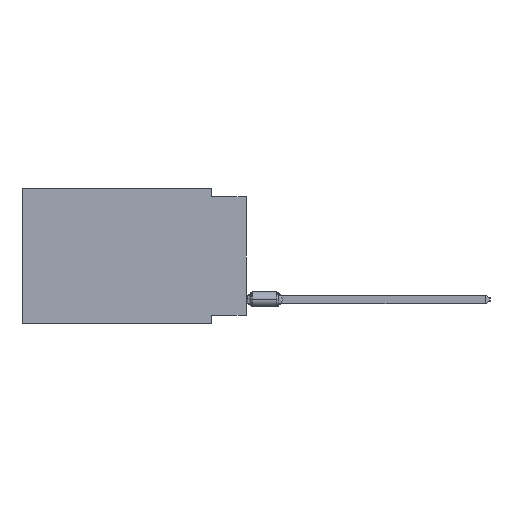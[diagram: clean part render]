
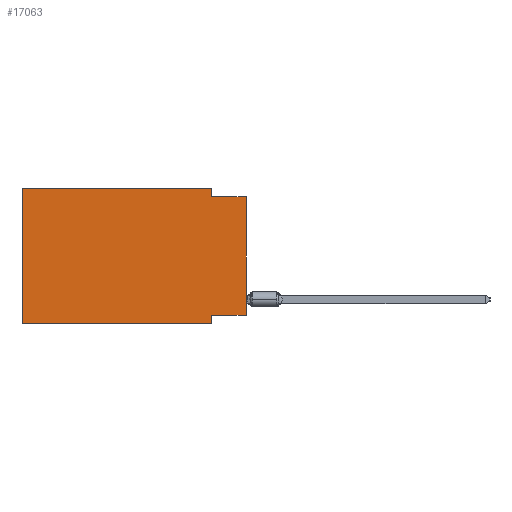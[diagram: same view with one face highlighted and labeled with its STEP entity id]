
A CAD part, left-side view. The second image highlights one B-rep face of the part: STEP entity #17063.
In plain terms, the highlighted planar face has unit normal (-1, 0, 0).
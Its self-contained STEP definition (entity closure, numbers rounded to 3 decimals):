
#175 = ORIENTED_EDGE ( 'NONE', *, *, #20337, .T. ) ;
#227 = CARTESIAN_POINT ( 'NONE',  ( 0., 2.54, 0. ) ) ;
#820 = LINE ( 'NONE', #16271, #21620 ) ;
#1589 = CARTESIAN_POINT ( 'NONE',  ( 0., 0., 0. ) ) ;
#2662 = CARTESIAN_POINT ( 'NONE',  ( 0., 16.383, 0. ) ) ;
#2813 = DIRECTION ( 'NONE',  ( 0., -1., 0. ) ) ;
#3084 = LINE ( 'NONE', #227, #20150 ) ;
#3428 = EDGE_LOOP ( 'NONE', ( #11187, #7930, #12192, #9831, #29777, #175, #21519, #31824 ) ) ;
#4492 = CARTESIAN_POINT ( 'NONE',  ( 0., 2.54, -0.635 ) ) ;
#5919 = DIRECTION ( 'NONE',  ( 0., 0., 1. ) ) ;
#6068 = LINE ( 'NONE', #15609, #21436 ) ;
#6574 = DIRECTION ( 'NONE',  ( 0., -1., 0. ) ) ;
#7838 = CARTESIAN_POINT ( 'NONE',  ( 0., 16.383, 0. ) ) ;
#7930 = ORIENTED_EDGE ( 'NONE', *, *, #35689, .F. ) ;
#8203 = VECTOR ( 'NONE', #6574, 1000. ) ;
#8391 = EDGE_CURVE ( 'NONE', #27628, #26745, #33743, .T. ) ;
#9180 = CARTESIAN_POINT ( 'NONE',  ( 0., 0., -9.271 ) ) ;
#9636 = LINE ( 'NONE', #22015, #8203 ) ;
#9831 = ORIENTED_EDGE ( 'NONE', *, *, #19126, .F. ) ;
#10632 = CARTESIAN_POINT ( 'NONE',  ( 0., 2.54, -9.906 ) ) ;
#11187 = ORIENTED_EDGE ( 'NONE', *, *, #39941, .T. ) ;
#11310 = PLANE ( 'NONE',  #29181 ) ;
#11545 = DIRECTION ( 'NONE',  ( 0., 0., -1. ) ) ;
#12192 = ORIENTED_EDGE ( 'NONE', *, *, #30972, .F. ) ;
#13540 = FACE_OUTER_BOUND ( 'NONE', #3428, .T. ) ;
#15276 = DIRECTION ( 'NONE',  ( 0., 0., -1. ) ) ;
#15609 = CARTESIAN_POINT ( 'NONE',  ( 0., 16.383, 0. ) ) ;
#15982 = EDGE_CURVE ( 'NONE', #39710, #19203, #22018, .T. ) ;
#16074 = VERTEX_POINT ( 'NONE', #36632 ) ;
#16271 = CARTESIAN_POINT ( 'NONE',  ( 0., 0., -0.635 ) ) ;
#16374 = VECTOR ( 'NONE', #5919, 1000. ) ;
#17063 = ADVANCED_FACE ( 'NONE', ( #13540 ), #11310, .F. ) ;
#17329 = VERTEX_POINT ( 'NONE', #4492 ) ;
#18979 = VERTEX_POINT ( 'NONE', #10632 ) ;
#19126 = EDGE_CURVE ( 'NONE', #26745, #16074, #6068, .T. ) ;
#19203 = VERTEX_POINT ( 'NONE', #38316 ) ;
#20150 = VECTOR ( 'NONE', #15276, 1000. ) ;
#20281 = DIRECTION ( 'NONE',  ( 0., 0., 1. ) ) ;
#20337 = EDGE_CURVE ( 'NONE', #27628, #18979, #9636, .T. ) ;
#20988 = CARTESIAN_POINT ( 'NONE',  ( 0., 16.383, -9.906 ) ) ;
#21436 = VECTOR ( 'NONE', #2813, 1000. ) ;
#21519 = ORIENTED_EDGE ( 'NONE', *, *, #37489, .F. ) ;
#21620 = VECTOR ( 'NONE', #22365, 1000. ) ;
#22015 = CARTESIAN_POINT ( 'NONE',  ( 0., 16.383, -9.906 ) ) ;
#22018 = LINE ( 'NONE', #37434, #31030 ) ;
#22365 = DIRECTION ( 'NONE',  ( 0., -1., 0. ) ) ;
#23530 = LINE ( 'NONE', #35469, #27085 ) ;
#24896 = DIRECTION ( 'NONE',  ( 0., 1., 0. ) ) ;
#25953 = DIRECTION ( 'NONE',  ( 1., 0., 0. ) ) ;
#26745 = VERTEX_POINT ( 'NONE', #31891 ) ;
#27085 = VECTOR ( 'NONE', #11545, 1000. ) ;
#27628 = VERTEX_POINT ( 'NONE', #20988 ) ;
#29181 = AXIS2_PLACEMENT_3D ( 'NONE', #7838, #25953, #38303 ) ;
#29777 = ORIENTED_EDGE ( 'NONE', *, *, #8391, .F. ) ;
#30972 = EDGE_CURVE ( 'NONE', #16074, #17329, #3084, .T. ) ;
#31030 = VECTOR ( 'NONE', #24896, 1000. ) ;
#31176 = VECTOR ( 'NONE', #20281, 1000. ) ;
#31264 = CARTESIAN_POINT ( 'NONE',  ( 0., 0., -0.635 ) ) ;
#31824 = ORIENTED_EDGE ( 'NONE', *, *, #15982, .F. ) ;
#31891 = CARTESIAN_POINT ( 'NONE',  ( 0., 16.383, 0. ) ) ;
#32864 = LINE ( 'NONE', #1589, #31176 ) ;
#33743 = LINE ( 'NONE', #2662, #16374 ) ;
#34989 = VERTEX_POINT ( 'NONE', #31264 ) ;
#35469 = CARTESIAN_POINT ( 'NONE',  ( 0., 2.54, -9.906 ) ) ;
#35689 = EDGE_CURVE ( 'NONE', #17329, #34989, #820, .T. ) ;
#36632 = CARTESIAN_POINT ( 'NONE',  ( 0., 2.54, 0. ) ) ;
#37434 = CARTESIAN_POINT ( 'NONE',  ( 0., 0., -9.271 ) ) ;
#37489 = EDGE_CURVE ( 'NONE', #19203, #18979, #23530, .T. ) ;
#38303 = DIRECTION ( 'NONE',  ( 0., 0., -1. ) ) ;
#38316 = CARTESIAN_POINT ( 'NONE',  ( 0., 2.54, -9.271 ) ) ;
#39710 = VERTEX_POINT ( 'NONE', #9180 ) ;
#39941 = EDGE_CURVE ( 'NONE', #39710, #34989, #32864, .T. ) ;
